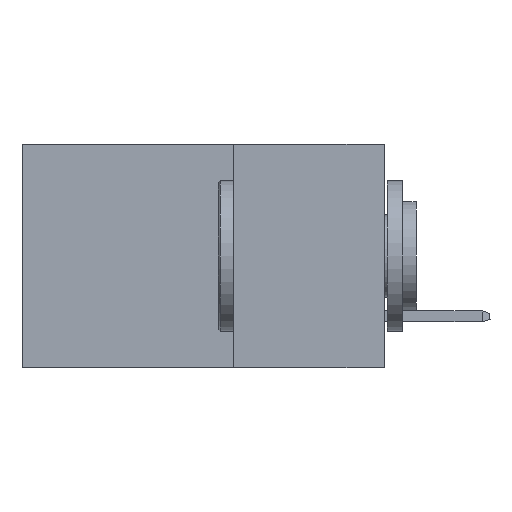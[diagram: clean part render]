
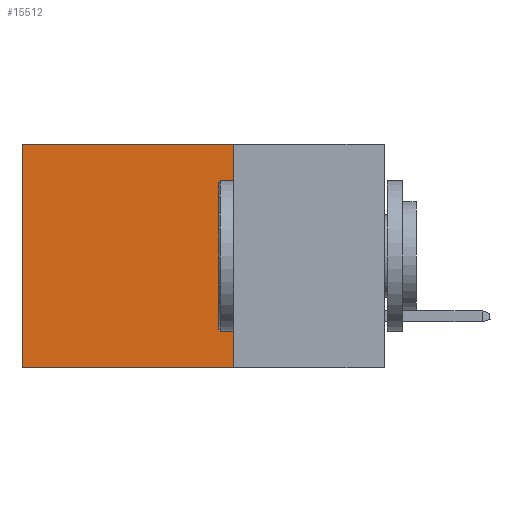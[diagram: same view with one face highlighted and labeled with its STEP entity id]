
A CAD part, left-side view. The second image highlights one B-rep face of the part: STEP entity #15512.
In plain terms, the highlighted planar face has unit normal (-1, 0, 0).
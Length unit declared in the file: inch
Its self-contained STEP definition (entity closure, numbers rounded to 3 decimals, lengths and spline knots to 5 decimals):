
#1726 = PLANE ( 'NONE',  #21062 ) ;
#2090 = LINE ( 'NONE', #16620, #14934 ) ;
#2876 = DIRECTION ( 'NONE',  ( 0., 1., 0. ) ) ;
#3092 = CARTESIAN_POINT ( 'NONE',  ( 0.298, 0.6, 0. ) ) ;
#6266 = VECTOR ( 'NONE', #21273, 39.37008 ) ;
#6622 = DIRECTION ( 'NONE',  ( 0., 1., 0. ) ) ;
#7267 = ORIENTED_EDGE ( 'NONE', *, *, #22292, .F. ) ;
#7504 = DIRECTION ( 'NONE',  ( 0., 0., -1. ) ) ;
#8142 = EDGE_CURVE ( 'NONE', #21061, #28419, #2090, .T. ) ;
#9029 = FACE_OUTER_BOUND ( 'NONE', #11099, .T. ) ;
#9135 = CARTESIAN_POINT ( 'NONE',  ( 0.298, 0.6, -0.37 ) ) ;
#9772 = ORIENTED_EDGE ( 'NONE', *, *, #10221, .T. ) ;
#10221 = EDGE_CURVE ( 'NONE', #28419, #25994, #24365, .T. ) ;
#10440 = DIRECTION ( 'NONE',  ( 1., 0., 0. ) ) ;
#11099 = EDGE_LOOP ( 'NONE', ( #9772, #7267, #27316, #25973 ) ) ;
#11189 = LINE ( 'NONE', #23478, #28606 ) ;
#11627 = VECTOR ( 'NONE', #6622, 39.37008 ) ;
#13402 = CARTESIAN_POINT ( 'NONE',  ( 0.298, 0.25, -0.37 ) ) ;
#13950 = CARTESIAN_POINT ( 'NONE',  ( 0.298, 0.6, 0. ) ) ;
#14934 = VECTOR ( 'NONE', #2876, 39.37008 ) ;
#15512 = ADVANCED_FACE ( 'NONE', ( #9029 ), #1726, .F. ) ;
#15968 = VERTEX_POINT ( 'NONE', #18127 ) ;
#16261 = LINE ( 'NONE', #13402, #11627 ) ;
#16617 = CARTESIAN_POINT ( 'NONE',  ( 0.298, 0.25, 0. ) ) ;
#16620 = CARTESIAN_POINT ( 'NONE',  ( 0.298, 0.25, 0. ) ) ;
#18127 = CARTESIAN_POINT ( 'NONE',  ( 0.298, 0.25, -0.37 ) ) ;
#21061 = VERTEX_POINT ( 'NONE', #16617 ) ;
#21062 = AXIS2_PLACEMENT_3D ( 'NONE', #24205, #10440, #29000 ) ;
#21273 = DIRECTION ( 'NONE',  ( 0., 0., -1. ) ) ;
#22292 = EDGE_CURVE ( 'NONE', #15968, #25994, #16261, .T. ) ;
#23478 = CARTESIAN_POINT ( 'NONE',  ( 0.298, 0.25, 0. ) ) ;
#24205 = CARTESIAN_POINT ( 'NONE',  ( 0.298, 0.25, 0. ) ) ;
#24365 = LINE ( 'NONE', #3092, #6266 ) ;
#25973 = ORIENTED_EDGE ( 'NONE', *, *, #8142, .T. ) ;
#25994 = VERTEX_POINT ( 'NONE', #9135 ) ;
#27316 = ORIENTED_EDGE ( 'NONE', *, *, #29162, .F. ) ;
#28419 = VERTEX_POINT ( 'NONE', #13950 ) ;
#28606 = VECTOR ( 'NONE', #7504, 39.37008 ) ;
#29000 = DIRECTION ( 'NONE',  ( 0., 0., -1. ) ) ;
#29162 = EDGE_CURVE ( 'NONE', #21061, #15968, #11189, .T. ) ;
